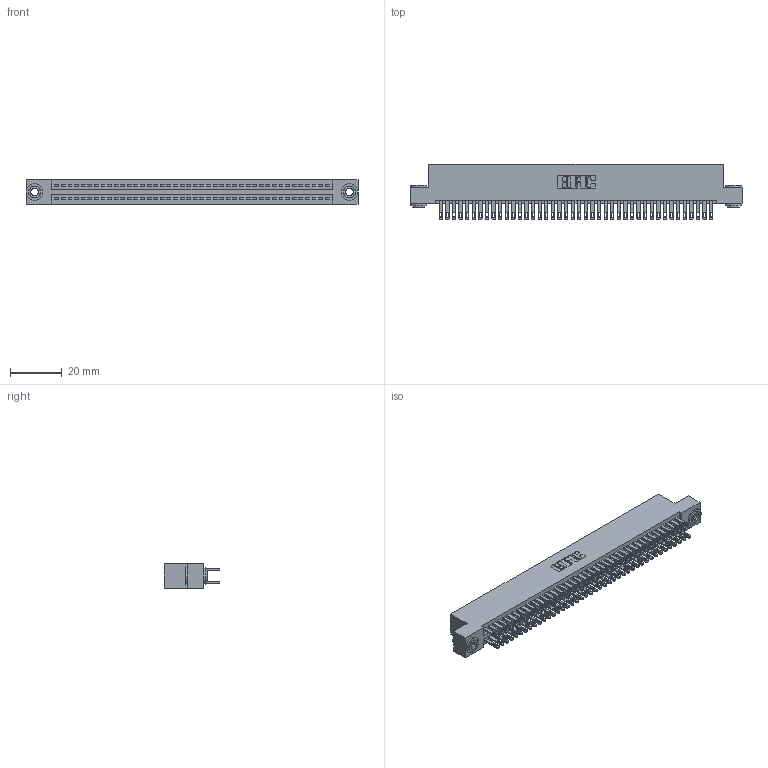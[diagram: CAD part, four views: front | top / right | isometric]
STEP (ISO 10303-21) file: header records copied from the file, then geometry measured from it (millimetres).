
FILE_DESCRIPTION (( 'STEP AP203' ), '1' );
FILE_NAME ('345-084-500-203.STEP', '2018-10-04T00:06:44', ( '' ), ( '' ), 'SwSTEP 2.0', 'SolidWorks 2016', '' );
FILE_SCHEMA (( 'CONFIG_CONTROL_DESIGN' ));
Length unit declared in the file: inch
Products named in the file (4): 345 Part_Flush Mounting Lugs - 0.156 Dia-TH; 345-250-002_345-250-002-102; 345-292-001_345-293-100; 345-084-500-203
Assembly tree (87 placements, depth 2):
  345-084-500-203
    345 Part_Flush Mounting Lugs - 0.156 Dia-TH
    345-292-001_345-293-100  x84
    345-250-002_345-250-002-102  x2
Bounding box: 127.89 x 21.51 x 9.4 mm (x, y, z)
Volume: 12699.4 mm3; surface area: 19833.4 mm2
Topology: 87 solids, 87 shells, 4028 faces, 12261 edges, 8170 vertices
Faces by surface type: plane 2358, cylinder 1662, cone 8
Entity records: 33534 total; most frequent: CARTESIAN_POINT 5595, ORIENTED_EDGE 5522, DIRECTION 4967, EDGE_CURVE 2761, VECTOR 2433, LINE 2433, VERTEX_POINT 1838, AXIS2_PLACEMENT_3D 1267
